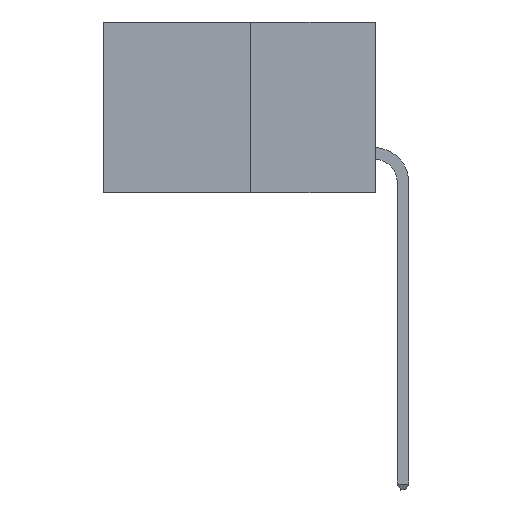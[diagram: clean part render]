
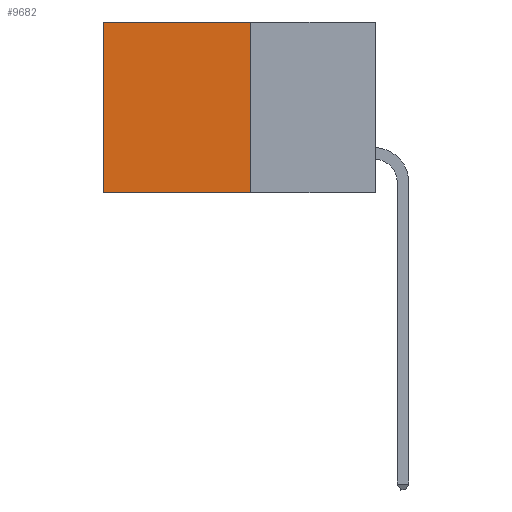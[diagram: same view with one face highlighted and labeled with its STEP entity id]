
A CAD part, left-side view. The second image highlights one B-rep face of the part: STEP entity #9682.
In plain terms, the highlighted planar face has unit normal (-1, 0, 0).
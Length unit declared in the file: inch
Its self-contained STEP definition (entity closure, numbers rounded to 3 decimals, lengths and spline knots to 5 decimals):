
#596 = VERTEX_POINT ( 'NONE', #18754 ) ;
#2334 = LINE ( 'NONE', #14870, #14987 ) ;
#2780 = ORIENTED_EDGE ( 'NONE', *, *, #4131, .F. ) ;
#3039 = LINE ( 'NONE', #7406, #7654 ) ;
#3727 = DIRECTION ( 'NONE',  ( 0., 1., 0. ) ) ;
#3844 = DIRECTION ( 'NONE',  ( 0., 1., 0. ) ) ;
#4131 = EDGE_CURVE ( 'NONE', #18080, #14007, #3039, .T. ) ;
#4930 = CARTESIAN_POINT ( 'NONE',  ( 0.277, 0.27, -0.37 ) ) ;
#5090 = EDGE_LOOP ( 'NONE', ( #9058, #2780, #11919, #9678 ) ) ;
#5376 = CARTESIAN_POINT ( 'NONE',  ( 0.277, 0.27, -0.37 ) ) ;
#5963 = AXIS2_PLACEMENT_3D ( 'NONE', #4930, #22023, #11887 ) ;
#7406 = CARTESIAN_POINT ( 'NONE',  ( 0.277, 0.27, -0.37 ) ) ;
#7654 = VECTOR ( 'NONE', #3844, 39.37008 ) ;
#9058 = ORIENTED_EDGE ( 'NONE', *, *, #15312, .T. ) ;
#9519 = LINE ( 'NONE', #17501, #14084 ) ;
#9678 = ORIENTED_EDGE ( 'NONE', *, *, #15631, .T. ) ;
#9682 = ADVANCED_FACE ( 'NONE', ( #12919 ), #10136, .F. ) ;
#10136 = PLANE ( 'NONE',  #5963 ) ;
#10888 = EDGE_CURVE ( 'NONE', #596, #18080, #2334, .T. ) ;
#11471 = DIRECTION ( 'NONE',  ( 0., 0., -1. ) ) ;
#11887 = DIRECTION ( 'NONE',  ( 0., 0., -1. ) ) ;
#11919 = ORIENTED_EDGE ( 'NONE', *, *, #10888, .F. ) ;
#12080 = CARTESIAN_POINT ( 'NONE',  ( 0.277, 0.59, 0. ) ) ;
#12919 = FACE_OUTER_BOUND ( 'NONE', #5090, .T. ) ;
#13293 = CARTESIAN_POINT ( 'NONE',  ( 0.277, 0.59, -0.37 ) ) ;
#13296 = CARTESIAN_POINT ( 'NONE',  ( 0.277, 0.59, -0.37 ) ) ;
#14007 = VERTEX_POINT ( 'NONE', #13296 ) ;
#14084 = VECTOR ( 'NONE', #3727, 39.37008 ) ;
#14870 = CARTESIAN_POINT ( 'NONE',  ( 0.277, 0.27, -0.37 ) ) ;
#14987 = VECTOR ( 'NONE', #11471, 39.37008 ) ;
#15023 = DIRECTION ( 'NONE',  ( 0., 0., -1. ) ) ;
#15312 = EDGE_CURVE ( 'NONE', #16745, #14007, #15890, .T. ) ;
#15631 = EDGE_CURVE ( 'NONE', #596, #16745, #9519, .T. ) ;
#15890 = LINE ( 'NONE', #13293, #16426 ) ;
#16426 = VECTOR ( 'NONE', #15023, 39.37008 ) ;
#16745 = VERTEX_POINT ( 'NONE', #12080 ) ;
#17501 = CARTESIAN_POINT ( 'NONE',  ( 0.277, 0.27, 0. ) ) ;
#18080 = VERTEX_POINT ( 'NONE', #5376 ) ;
#18754 = CARTESIAN_POINT ( 'NONE',  ( 0.277, 0.27, 0. ) ) ;
#22023 = DIRECTION ( 'NONE',  ( 1., 0., 0. ) ) ;
